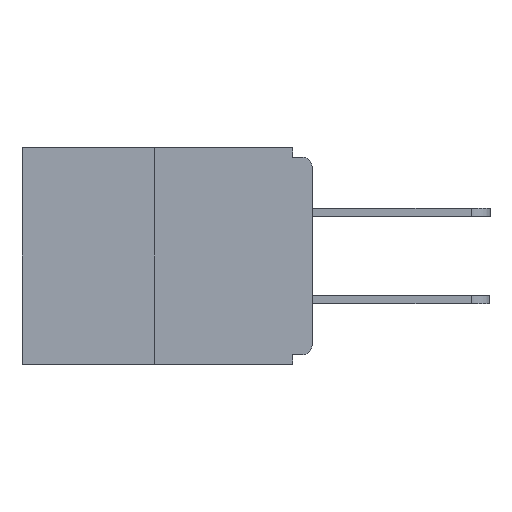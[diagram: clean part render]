
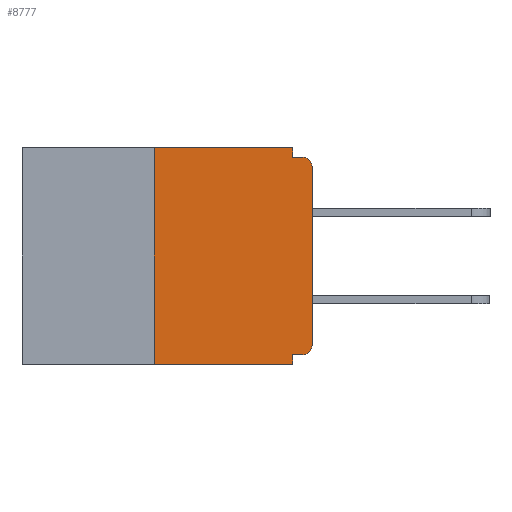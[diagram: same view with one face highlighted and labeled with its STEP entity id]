
A CAD part, left-side view. The second image highlights one B-rep face of the part: STEP entity #8777.
In plain terms, the highlighted planar face has unit normal (-1, 0, 0).
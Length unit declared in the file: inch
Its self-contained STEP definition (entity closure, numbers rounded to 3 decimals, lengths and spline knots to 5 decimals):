
#150 = AXIS2_PLACEMENT_3D ( 'NONE', #12463, #16523, #6700 ) ;
#199 = DIRECTION ( 'NONE',  ( 0., 0., -1. ) ) ;
#673 = EDGE_CURVE ( 'NONE', #2635, #10329, #17007, .T. ) ;
#1180 = LINE ( 'NONE', #2115, #6747 ) ;
#1202 = FACE_OUTER_BOUND ( 'NONE', #13699, .T. ) ;
#1330 = ORIENTED_EDGE ( 'NONE', *, *, #6921, .F. ) ;
#1645 = CIRCLE ( 'NONE', #5687, 0.015 ) ;
#1792 = PLANE ( 'NONE',  #16944 ) ;
#1794 = CARTESIAN_POINT ( 'NONE',  ( 0., 0.46, 0. ) ) ;
#1832 = CARTESIAN_POINT ( 'NONE',  ( 0., 0.031, -0.343 ) ) ;
#1878 = VECTOR ( 'NONE', #2311, 39.37008 ) ;
#1931 = DIRECTION ( 'NONE',  ( 0., 0., 1. ) ) ;
#2098 = CARTESIAN_POINT ( 'NONE',  ( 0., 0.25, 0. ) ) ;
#2115 = CARTESIAN_POINT ( 'NONE',  ( 0., 0.25, 0. ) ) ;
#2194 = CARTESIAN_POINT ( 'NONE',  ( 0., 0.46, -0.343 ) ) ;
#2311 = DIRECTION ( 'NONE',  ( 0., -1., 0. ) ) ;
#2348 = EDGE_CURVE ( 'NONE', #13712, #12937, #14968, .T. ) ;
#2372 = CARTESIAN_POINT ( 'NONE',  ( 0., 0., -0.03 ) ) ;
#2476 = CARTESIAN_POINT ( 'NONE',  ( 0., 0., -0.015 ) ) ;
#2635 = VERTEX_POINT ( 'NONE', #6248 ) ;
#3653 = VECTOR ( 'NONE', #199, 39.37008 ) ;
#3734 = LINE ( 'NONE', #1832, #16595 ) ;
#4150 = VERTEX_POINT ( 'NONE', #4923 ) ;
#4152 = LINE ( 'NONE', #1794, #7862 ) ;
#4167 = ORIENTED_EDGE ( 'NONE', *, *, #673, .T. ) ;
#4735 = CARTESIAN_POINT ( 'NONE',  ( 0., 0.031, -0.343 ) ) ;
#4754 = DIRECTION ( 'NONE',  ( 1., 0., 0. ) ) ;
#4887 = DIRECTION ( 'NONE',  ( 0., 0., 1. ) ) ;
#4919 = EDGE_CURVE ( 'NONE', #14163, #6201, #15177, .T. ) ;
#4923 = CARTESIAN_POINT ( 'NONE',  ( 0., 0.015, -0.015 ) ) ;
#5501 = DIRECTION ( 'NONE',  ( -1., 0., 0. ) ) ;
#5561 = DIRECTION ( 'NONE',  ( 0., 0., -1. ) ) ;
#5687 = AXIS2_PLACEMENT_3D ( 'NONE', #15260, #5501, #5561 ) ;
#5845 = CARTESIAN_POINT ( 'NONE',  ( 0., 0.031, 0. ) ) ;
#6201 = VERTEX_POINT ( 'NONE', #14508 ) ;
#6248 = CARTESIAN_POINT ( 'NONE',  ( 0., 0., -0.313 ) ) ;
#6700 = DIRECTION ( 'NONE',  ( 0., 0., -1. ) ) ;
#6747 = VECTOR ( 'NONE', #1931, 39.37008 ) ;
#6921 = EDGE_CURVE ( 'NONE', #8389, #12937, #3734, .T. ) ;
#7118 = ORIENTED_EDGE ( 'NONE', *, *, #12434, .F. ) ;
#7862 = VECTOR ( 'NONE', #15755, 39.37008 ) ;
#7922 = ORIENTED_EDGE ( 'NONE', *, *, #2348, .T. ) ;
#7991 = ORIENTED_EDGE ( 'NONE', *, *, #8185, .F. ) ;
#8185 = EDGE_CURVE ( 'NONE', #14881, #8389, #17528, .T. ) ;
#8214 = ORIENTED_EDGE ( 'NONE', *, *, #13075, .T. ) ;
#8389 = VERTEX_POINT ( 'NONE', #17557 ) ;
#8777 = ADVANCED_FACE ( 'NONE', ( #1202 ), #1792, .F. ) ;
#8908 = ORIENTED_EDGE ( 'NONE', *, *, #4919, .F. ) ;
#9801 = VECTOR ( 'NONE', #11978, 39.37008 ) ;
#9815 = VERTEX_POINT ( 'NONE', #2098 ) ;
#10329 = VERTEX_POINT ( 'NONE', #2372 ) ;
#10471 = CARTESIAN_POINT ( 'NONE',  ( 0., 0.031, 0. ) ) ;
#10543 = EDGE_CURVE ( 'NONE', #13712, #9815, #1180, .T. ) ;
#10808 = ORIENTED_EDGE ( 'NONE', *, *, #10543, .F. ) ;
#11978 = DIRECTION ( 'NONE',  ( 0., -1., 0. ) ) ;
#11980 = VECTOR ( 'NONE', #4887, 39.37008 ) ;
#12265 = CARTESIAN_POINT ( 'NONE',  ( 0., 0.25, -0.343 ) ) ;
#12434 = EDGE_CURVE ( 'NONE', #6201, #4150, #16745, .T. ) ;
#12463 = CARTESIAN_POINT ( 'NONE',  ( 0., 0.015, -0.03 ) ) ;
#12632 = CARTESIAN_POINT ( 'NONE',  ( 0., 0.015, -0.328 ) ) ;
#12888 = ORIENTED_EDGE ( 'NONE', *, *, #17608, .T. ) ;
#12937 = VERTEX_POINT ( 'NONE', #4735 ) ;
#13043 = DIRECTION ( 'NONE',  ( 0., 0., -1. ) ) ;
#13075 = EDGE_CURVE ( 'NONE', #14881, #2635, #1645, .T. ) ;
#13174 = CARTESIAN_POINT ( 'NONE',  ( 0., 0.46, 0. ) ) ;
#13699 = EDGE_LOOP ( 'NONE', ( #14935, #10808, #7922, #1330, #7991, #8214, #4167, #12888, #7118, #8908 ) ) ;
#13712 = VERTEX_POINT ( 'NONE', #12265 ) ;
#13845 = VECTOR ( 'NONE', #17438, 39.37008 ) ;
#14163 = VERTEX_POINT ( 'NONE', #10471 ) ;
#14361 = DIRECTION ( 'NONE',  ( 0., 0., -1. ) ) ;
#14508 = CARTESIAN_POINT ( 'NONE',  ( 0., 0.031, -0.015 ) ) ;
#14881 = VERTEX_POINT ( 'NONE', #12632 ) ;
#14935 = ORIENTED_EDGE ( 'NONE', *, *, #17745, .F. ) ;
#14968 = LINE ( 'NONE', #2194, #9801 ) ;
#15177 = LINE ( 'NONE', #5845, #3653 ) ;
#15260 = CARTESIAN_POINT ( 'NONE',  ( 0., 0.015, -0.313 ) ) ;
#15755 = DIRECTION ( 'NONE',  ( 0., -1., 0. ) ) ;
#15894 = CARTESIAN_POINT ( 'NONE',  ( 0., 0., 0. ) ) ;
#16523 = DIRECTION ( 'NONE',  ( -1., 0., 0. ) ) ;
#16577 = CIRCLE ( 'NONE', #150, 0.015 ) ;
#16595 = VECTOR ( 'NONE', #13043, 39.37008 ) ;
#16745 = LINE ( 'NONE', #2476, #1878 ) ;
#16944 = AXIS2_PLACEMENT_3D ( 'NONE', #13174, #4754, #14361 ) ;
#17007 = LINE ( 'NONE', #15894, #11980 ) ;
#17438 = DIRECTION ( 'NONE',  ( 0., 1., 0. ) ) ;
#17491 = CARTESIAN_POINT ( 'NONE',  ( 0., 0., -0.328 ) ) ;
#17528 = LINE ( 'NONE', #17491, #13845 ) ;
#17557 = CARTESIAN_POINT ( 'NONE',  ( 0., 0.031, -0.328 ) ) ;
#17608 = EDGE_CURVE ( 'NONE', #10329, #4150, #16577, .T. ) ;
#17745 = EDGE_CURVE ( 'NONE', #9815, #14163, #4152, .T. ) ;
